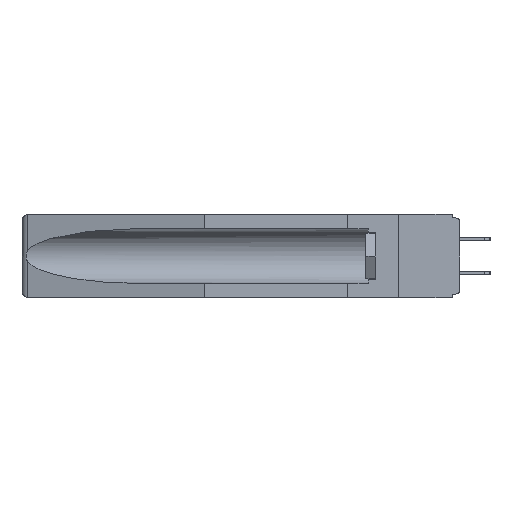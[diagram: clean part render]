
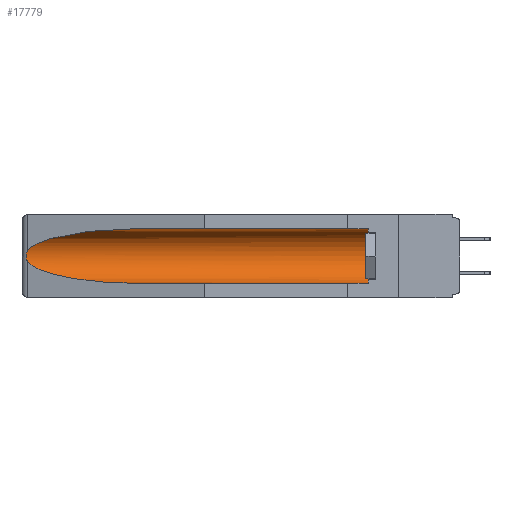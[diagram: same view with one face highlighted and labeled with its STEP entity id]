
A CAD part, left-side view. The second image highlights one B-rep face of the part: STEP entity #17779.
In plain terms, the highlighted cylindrical face has radius 2.857 mm (diameter 5.715 mm), a partial arc.
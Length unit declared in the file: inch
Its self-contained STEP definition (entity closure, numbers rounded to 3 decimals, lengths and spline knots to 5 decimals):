
#170 = DIRECTION ( 'NONE',  ( 0., 1., 0. ) ) ;
#533 = CARTESIAN_POINT ( 'NONE',  ( 0.26537, 1.52718, -0.14972 ) ) ;
#1023 = CARTESIAN_POINT ( 'NONE',  ( 0.2673, 1.5327, -0.16383 ) ) ;
#1618 = CARTESIAN_POINT ( 'NONE',  ( 0.21114, 1.30732, -0.059 ) ) ;
#1777 = VERTEX_POINT ( 'NONE', #18553 ) ;
#1850 = CARTESIAN_POINT ( 'NONE',  ( 0.155, 0.126, -0.059 ) ) ;
#2012 = ORIENTED_EDGE ( 'NONE', *, *, #3345, .T. ) ;
#2616 = AXIS2_PLACEMENT_3D ( 'NONE', #11989, #2808, #17485 ) ;
#2717 = EDGE_LOOP ( 'NONE', ( #23036, #17276, #8871, #13484, #20428, #2012 ) ) ;
#2759 = EDGE_CURVE ( 'NONE', #16261, #18020, #13574, .T. ) ;
#2808 = DIRECTION ( 'NONE',  ( 0., -1., 0. ) ) ;
#2877 = CARTESIAN_POINT ( 'NONE',  ( 0.26655, 1.53094, -0.18657 ) ) ;
#3345 = EDGE_CURVE ( 'NONE', #8612, #12734, #5782, .T. ) ;
#3391 = VERTEX_POINT ( 'NONE', #533 ) ;
#3452 = CARTESIAN_POINT ( 'NONE',  ( 0.26537, 1.52718, -0.14972 ) ) ;
#4193 = CARTESIAN_POINT ( 'NONE',  ( 0.25451, 1.48313, -0.24835 ) ) ;
#4228 = LINE ( 'NONE', #13162, #23186 ) ;
#5517 = CARTESIAN_POINT ( 'NONE',  ( 0.26537, 1.52718, -0.19328 ) ) ;
#5769 = DIRECTION ( 'NONE',  ( 0., 1., 0. ) ) ;
#5782 = LINE ( 'NONE', #9417, #23298 ) ;
#6264 = CARTESIAN_POINT ( 'NONE',  ( 0.2673, 1.53269, -0.17917 ) ) ;
#7164 = CARTESIAN_POINT ( 'NONE',  ( 0.155, 1.07973, -0.059 ) ) ;
#7670 = CARTESIAN_POINT ( 'NONE',  ( 0.155, 1.07973, -0.284 ) ) ;
#7953 = CYLINDRICAL_SURFACE ( 'NONE', #18441, 0.1125 ) ;
#8612 = VERTEX_POINT ( 'NONE', #1850 ) ;
#8871 = ORIENTED_EDGE ( 'NONE', *, *, #2759, .T. ) ;
#8989 = CARTESIAN_POINT ( 'NONE',  ( 0.155, 1.07973, -0.284 ) ) ;
#9417 = CARTESIAN_POINT ( 'NONE',  ( 0.155, -0.30754, -0.059 ) ) ;
#10810 = B_SPLINE_CURVE_WITH_KNOTS ( 'NONE', 3,
 ( #17469, #21180, #12051, #1023, #13874, #17232, #6264, #2877, #15723, #21344 ),
 .UNSPECIFIED., .F., .F.,
 ( 4, 2, 2, 2, 4 ),
 ( 0., 0.00029, 0.00058, 0.00087, 0.00117 ),
 .UNSPECIFIED. ) ;
#11279 = CARTESIAN_POINT ( 'NONE',  ( 0.21114, 1.30732, -0.284 ) ) ;
#11989 = CARTESIAN_POINT ( 'NONE',  ( 0.155, 0.126, -0.1715 ) ) ;
#12051 = CARTESIAN_POINT ( 'NONE',  ( 0.26654, 1.53092, -0.15636 ) ) ;
#12734 = VERTEX_POINT ( 'NONE', #22850 ) ;
#13127 = EDGE_CURVE ( 'NONE', #1777, #8612, #17107, .T. ) ;
#13162 = CARTESIAN_POINT ( 'NONE',  ( 0.155, -0.30754, -0.284 ) ) ;
#13484 = ORIENTED_EDGE ( 'NONE', *, *, #17034, .F. ) ;
#13574 =( BOUNDED_CURVE ( )  B_SPLINE_CURVE ( 3, ( #5517, #4193, #11279, #7670 ),
 .UNSPECIFIED., .F., .F. ) 
 B_SPLINE_CURVE_WITH_KNOTS ( ( 4, 4 ),
 ( 0.1948, 1.5708 ),
 .UNSPECIFIED. ) 
 CURVE ( )  GEOMETRIC_REPRESENTATION_ITEM ( )  RATIONAL_B_SPLINE_CURVE ( ( 1., 0.848, 0.848, 1. ) ) 
 REPRESENTATION_ITEM ( '' )  );
#13874 = CARTESIAN_POINT ( 'NONE',  ( 0.2675, 1.53308, -0.16763 ) ) ;
#14447 = CARTESIAN_POINT ( 'NONE',  ( 0.25451, 1.48313, -0.09465 ) ) ;
#15090 = CARTESIAN_POINT ( 'NONE',  ( 0.155, -0.30754, -0.1715 ) ) ;
#15304 = DIRECTION ( 'NONE',  ( 0., 1., 0. ) ) ;
#15723 = CARTESIAN_POINT ( 'NONE',  ( 0.26597, 1.5296, -0.19026 ) ) ;
#16261 = VERTEX_POINT ( 'NONE', #17540 ) ;
#17034 = EDGE_CURVE ( 'NONE', #1777, #18020, #4228, .T. ) ;
#17091 =( BOUNDED_CURVE ( )  B_SPLINE_CURVE ( 3, ( #7164, #1618, #14447, #3452 ),
 .UNSPECIFIED., .F., .F. ) 
 B_SPLINE_CURVE_WITH_KNOTS ( ( 4, 4 ),
 ( 4.71239, 6.08839 ),
 .UNSPECIFIED. ) 
 CURVE ( )  GEOMETRIC_REPRESENTATION_ITEM ( )  RATIONAL_B_SPLINE_CURVE ( ( 1., 0.848, 0.848, 1. ) ) 
 REPRESENTATION_ITEM ( '' )  );
#17107 = CIRCLE ( 'NONE', #2616, 0.1125 ) ;
#17232 = CARTESIAN_POINT ( 'NONE',  ( 0.2675, 1.53308, -0.17534 ) ) ;
#17276 = ORIENTED_EDGE ( 'NONE', *, *, #19196, .T. ) ;
#17469 = CARTESIAN_POINT ( 'NONE',  ( 0.26537, 1.52718, -0.14972 ) ) ;
#17485 = DIRECTION ( 'NONE',  ( 0., 0., 1. ) ) ;
#17540 = CARTESIAN_POINT ( 'NONE',  ( 0.26537, 1.52718, -0.19328 ) ) ;
#17779 = ADVANCED_FACE ( 'NONE', ( #23760 ), #7953, .F. ) ;
#18020 = VERTEX_POINT ( 'NONE', #8989 ) ;
#18127 = EDGE_CURVE ( 'NONE', #12734, #3391, #17091, .T. ) ;
#18441 = AXIS2_PLACEMENT_3D ( 'NONE', #15090, #15304, #18675 ) ;
#18553 = CARTESIAN_POINT ( 'NONE',  ( 0.155, 0.126, -0.284 ) ) ;
#18675 = DIRECTION ( 'NONE',  ( 0., 0., 1. ) ) ;
#19196 = EDGE_CURVE ( 'NONE', #3391, #16261, #10810, .T. ) ;
#20428 = ORIENTED_EDGE ( 'NONE', *, *, #13127, .T. ) ;
#21180 = CARTESIAN_POINT ( 'NONE',  ( 0.26597, 1.52961, -0.15275 ) ) ;
#21344 = CARTESIAN_POINT ( 'NONE',  ( 0.26537, 1.52718, -0.19328 ) ) ;
#22850 = CARTESIAN_POINT ( 'NONE',  ( 0.155, 1.07973, -0.059 ) ) ;
#23036 = ORIENTED_EDGE ( 'NONE', *, *, #18127, .T. ) ;
#23186 = VECTOR ( 'NONE', #5769, 39.37008 ) ;
#23298 = VECTOR ( 'NONE', #170, 39.37008 ) ;
#23760 = FACE_OUTER_BOUND ( 'NONE', #2717, .T. ) ;
